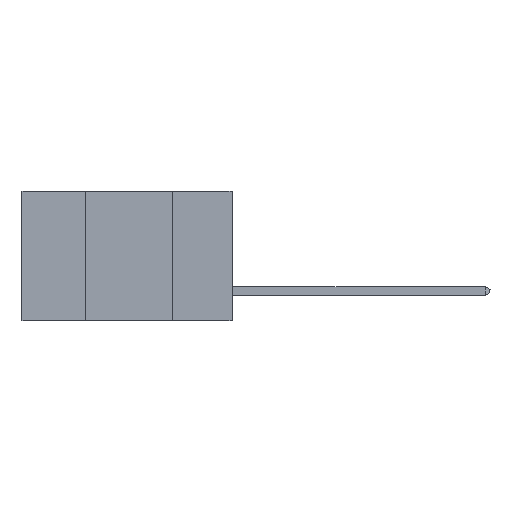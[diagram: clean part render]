
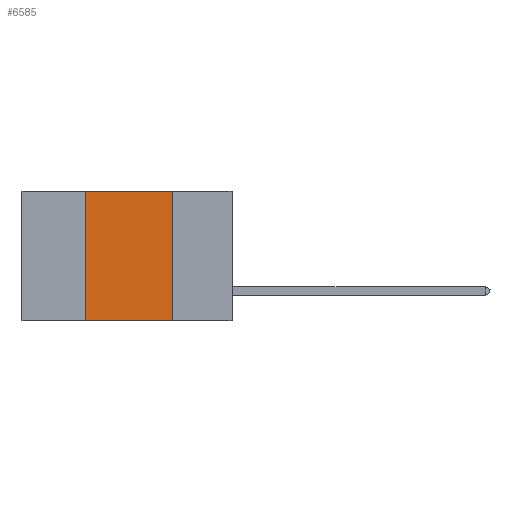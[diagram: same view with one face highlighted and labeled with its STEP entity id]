
A CAD part, left-side view. The second image highlights one B-rep face of the part: STEP entity #6585.
In plain terms, the highlighted planar face has unit normal (-1, 0, 0).
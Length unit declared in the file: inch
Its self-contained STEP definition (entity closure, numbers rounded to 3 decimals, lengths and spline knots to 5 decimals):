
#425 = EDGE_CURVE ( 'NONE', #8401, #15542, #918, .T. ) ;
#918 = LINE ( 'NONE', #20007, #5354 ) ;
#1842 = EDGE_CURVE ( 'NONE', #18571, #15542, #6000, .T. ) ;
#2791 = DIRECTION ( 'NONE',  ( 0., -1., 0. ) ) ;
#3940 = ORIENTED_EDGE ( 'NONE', *, *, #8161, .F. ) ;
#5354 = VECTOR ( 'NONE', #2791, 39.37008 ) ;
#5477 = VECTOR ( 'NONE', #12773, 39.37008 ) ;
#6000 = LINE ( 'NONE', #6474, #11416 ) ;
#6474 = CARTESIAN_POINT ( 'NONE',  ( 0., 0.17, 0. ) ) ;
#6585 = ADVANCED_FACE ( 'NONE', ( #12426 ), #8692, .F. ) ;
#6953 = LINE ( 'NONE', #7130, #10168 ) ;
#7130 = CARTESIAN_POINT ( 'NONE',  ( 0., 0.42, 0. ) ) ;
#7141 = DIRECTION ( 'NONE',  ( 1., 0., 0. ) ) ;
#7199 = DIRECTION ( 'NONE',  ( 0., 0., -1. ) ) ;
#7319 = CARTESIAN_POINT ( 'NONE',  ( 0., 0.42, -0.37 ) ) ;
#7510 = ORIENTED_EDGE ( 'NONE', *, *, #1842, .F. ) ;
#8161 = EDGE_CURVE ( 'NONE', #8401, #9429, #6953, .T. ) ;
#8401 = VERTEX_POINT ( 'NONE', #7319 ) ;
#8474 = EDGE_CURVE ( 'NONE', #9429, #18571, #19534, .T. ) ;
#8692 = PLANE ( 'NONE',  #18840 ) ;
#9429 = VERTEX_POINT ( 'NONE', #19071 ) ;
#10168 = VECTOR ( 'NONE', #20068, 39.37008 ) ;
#11416 = VECTOR ( 'NONE', #7199, 39.37008 ) ;
#11564 = CARTESIAN_POINT ( 'NONE',  ( 0., 0.17, 0. ) ) ;
#12426 = FACE_OUTER_BOUND ( 'NONE', #17509, .T. ) ;
#12441 = ORIENTED_EDGE ( 'NONE', *, *, #425, .T. ) ;
#12773 = DIRECTION ( 'NONE',  ( 0., -1., 0. ) ) ;
#15542 = VERTEX_POINT ( 'NONE', #15615 ) ;
#15615 = CARTESIAN_POINT ( 'NONE',  ( 0., 0.17, -0.37 ) ) ;
#15874 = CARTESIAN_POINT ( 'NONE',  ( 0., 0.6, 0. ) ) ;
#17320 = ORIENTED_EDGE ( 'NONE', *, *, #8474, .F. ) ;
#17509 = EDGE_LOOP ( 'NONE', ( #7510, #17320, #3940, #12441 ) ) ;
#18571 = VERTEX_POINT ( 'NONE', #11564 ) ;
#18840 = AXIS2_PLACEMENT_3D ( 'NONE', #19706, #7141, #19779 ) ;
#19071 = CARTESIAN_POINT ( 'NONE',  ( 0., 0.42, 0. ) ) ;
#19534 = LINE ( 'NONE', #15874, #5477 ) ;
#19706 = CARTESIAN_POINT ( 'NONE',  ( 0., 0.6, 0. ) ) ;
#19779 = DIRECTION ( 'NONE',  ( 0., 0., -1. ) ) ;
#20007 = CARTESIAN_POINT ( 'NONE',  ( 0., 0.6, -0.37 ) ) ;
#20068 = DIRECTION ( 'NONE',  ( 0., 0., 1. ) ) ;
